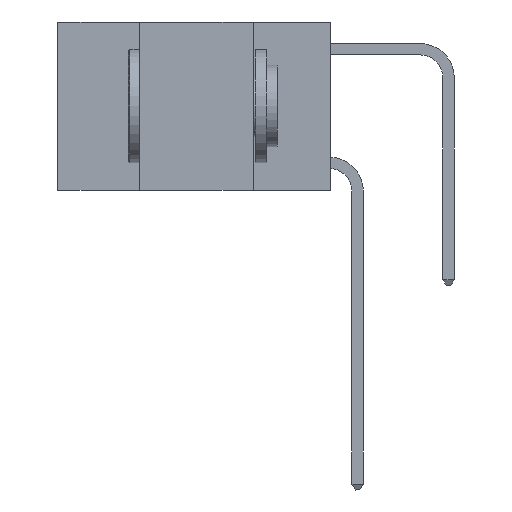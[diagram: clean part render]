
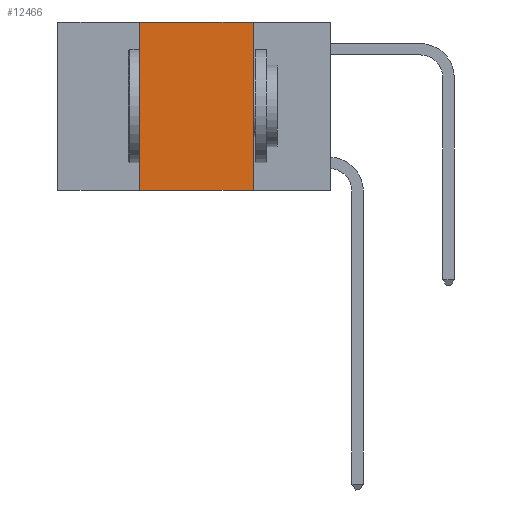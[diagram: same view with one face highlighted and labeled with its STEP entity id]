
A CAD part, left-side view. The second image highlights one B-rep face of the part: STEP entity #12466.
In plain terms, the highlighted planar face has unit normal (-1, 0, 0).
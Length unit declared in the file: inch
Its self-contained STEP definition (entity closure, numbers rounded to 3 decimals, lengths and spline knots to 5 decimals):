
#1522 = VERTEX_POINT ( 'NONE', #5794 ) ;
#1537 = EDGE_CURVE ( 'NONE', #10308, #1522, #3293, .T. ) ;
#1766 = EDGE_LOOP ( 'NONE', ( #10193, #11108, #4571, #3785 ) ) ;
#3167 = CARTESIAN_POINT ( 'NONE',  ( 0., 0.17, 0. ) ) ;
#3293 = LINE ( 'NONE', #10114, #12170 ) ;
#3785 = ORIENTED_EDGE ( 'NONE', *, *, #5990, .T. ) ;
#4069 = CARTESIAN_POINT ( 'NONE',  ( 0., 0.6, 0. ) ) ;
#4205 = VERTEX_POINT ( 'NONE', #12579 ) ;
#4571 = ORIENTED_EDGE ( 'NONE', *, *, #1537, .F. ) ;
#5222 = LINE ( 'NONE', #3167, #7530 ) ;
#5794 = CARTESIAN_POINT ( 'NONE',  ( 0., 0.42, 0. ) ) ;
#5804 = CARTESIAN_POINT ( 'NONE',  ( 0., 0.6, 0. ) ) ;
#5867 = LINE ( 'NONE', #4069, #7348 ) ;
#5868 = DIRECTION ( 'NONE',  ( 0., 0., -1. ) ) ;
#5990 = EDGE_CURVE ( 'NONE', #10308, #4205, #9103, .T. ) ;
#6850 = DIRECTION ( 'NONE',  ( 1., 0., 0. ) ) ;
#7130 = DIRECTION ( 'NONE',  ( 0., -1., 0. ) ) ;
#7246 = VERTEX_POINT ( 'NONE', #9362 ) ;
#7311 = VECTOR ( 'NONE', #7130, 39.37008 ) ;
#7348 = VECTOR ( 'NONE', #12016, 39.37008 ) ;
#7530 = VECTOR ( 'NONE', #8189, 39.37008 ) ;
#8189 = DIRECTION ( 'NONE',  ( 0., 0., -1. ) ) ;
#8829 = FACE_OUTER_BOUND ( 'NONE', #1766, .T. ) ;
#9069 = DIRECTION ( 'NONE',  ( 0., 0., 1. ) ) ;
#9103 = LINE ( 'NONE', #9943, #7311 ) ;
#9183 = AXIS2_PLACEMENT_3D ( 'NONE', #5804, #6850, #5868 ) ;
#9326 = EDGE_CURVE ( 'NONE', #7246, #4205, #5222, .T. ) ;
#9362 = CARTESIAN_POINT ( 'NONE',  ( 0., 0.17, 0. ) ) ;
#9396 = CARTESIAN_POINT ( 'NONE',  ( 0., 0.42, -0.37 ) ) ;
#9943 = CARTESIAN_POINT ( 'NONE',  ( 0., 0.6, -0.37 ) ) ;
#10114 = CARTESIAN_POINT ( 'NONE',  ( 0., 0.42, 0. ) ) ;
#10193 = ORIENTED_EDGE ( 'NONE', *, *, #9326, .F. ) ;
#10308 = VERTEX_POINT ( 'NONE', #9396 ) ;
#10641 = EDGE_CURVE ( 'NONE', #1522, #7246, #5867, .T. ) ;
#11108 = ORIENTED_EDGE ( 'NONE', *, *, #10641, .F. ) ;
#12016 = DIRECTION ( 'NONE',  ( 0., -1., 0. ) ) ;
#12170 = VECTOR ( 'NONE', #9069, 39.37008 ) ;
#12466 = ADVANCED_FACE ( 'NONE', ( #8829 ), #12734, .F. ) ;
#12579 = CARTESIAN_POINT ( 'NONE',  ( 0., 0.17, -0.37 ) ) ;
#12734 = PLANE ( 'NONE',  #9183 ) ;
